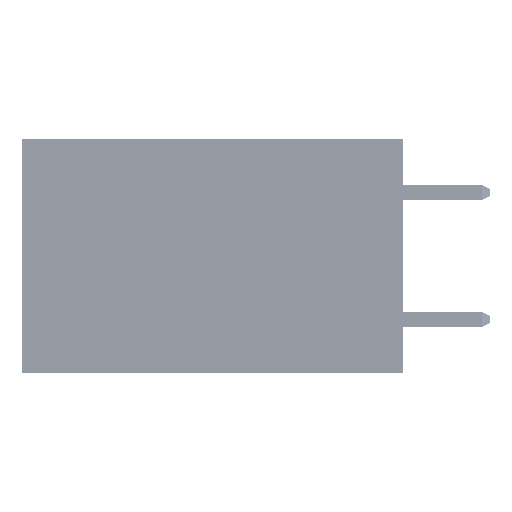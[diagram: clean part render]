
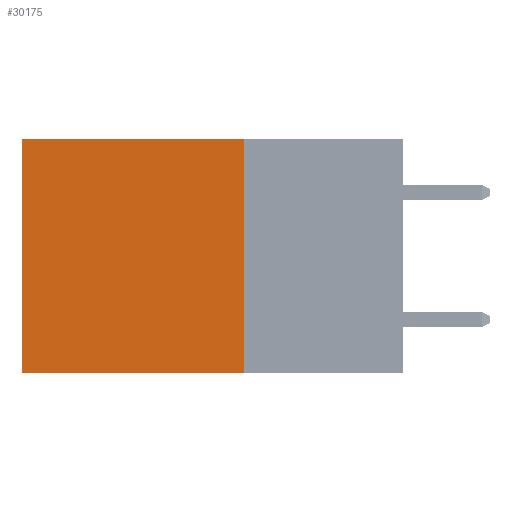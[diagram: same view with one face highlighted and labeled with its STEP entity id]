
A CAD part, left-side view. The second image highlights one B-rep face of the part: STEP entity #30175.
In plain terms, the highlighted planar face has unit normal (-1, 0, 0).
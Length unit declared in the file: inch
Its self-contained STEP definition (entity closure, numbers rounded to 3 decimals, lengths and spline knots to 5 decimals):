
#107 = ORIENTED_EDGE ( 'NONE', *, *, #25879, .F. ) ;
#2100 = CARTESIAN_POINT ( 'NONE',  ( 0.2875, 0.25, 0. ) ) ;
#3534 = VECTOR ( 'NONE', #37417, 39.37008 ) ;
#4212 = VECTOR ( 'NONE', #29039, 39.37008 ) ;
#8453 = CARTESIAN_POINT ( 'NONE',  ( 0.2875, 0.25, 0. ) ) ;
#9466 = AXIS2_PLACEMENT_3D ( 'NONE', #8453, #27998, #39258 ) ;
#11330 = VERTEX_POINT ( 'NONE', #11415 ) ;
#11401 = VERTEX_POINT ( 'NONE', #26607 ) ;
#11415 = CARTESIAN_POINT ( 'NONE',  ( 0.2875, 0.6, 0. ) ) ;
#12423 = EDGE_CURVE ( 'NONE', #17834, #11330, #48236, .T. ) ;
#12526 = CARTESIAN_POINT ( 'NONE',  ( 0.2875, 0.25, -0.37 ) ) ;
#13076 = VERTEX_POINT ( 'NONE', #12526 ) ;
#13215 = EDGE_CURVE ( 'NONE', #11330, #11401, #39036, .T. ) ;
#14314 = DIRECTION ( 'NONE',  ( 0., 0., -1. ) ) ;
#15822 = CARTESIAN_POINT ( 'NONE',  ( 0.2875, 0.25, -0.37 ) ) ;
#17834 = VERTEX_POINT ( 'NONE', #34041 ) ;
#19723 = LINE ( 'NONE', #49235, #35392 ) ;
#19757 = PLANE ( 'NONE',  #9466 ) ;
#19810 = FACE_OUTER_BOUND ( 'NONE', #33531, .T. ) ;
#24456 = ORIENTED_EDGE ( 'NONE', *, *, #12423, .T. ) ;
#25698 = ORIENTED_EDGE ( 'NONE', *, *, #13215, .T. ) ;
#25879 = EDGE_CURVE ( 'NONE', #13076, #11401, #29093, .T. ) ;
#26607 = CARTESIAN_POINT ( 'NONE',  ( 0.2875, 0.6, -0.37 ) ) ;
#27998 = DIRECTION ( 'NONE',  ( 1., 0., 0. ) ) ;
#29039 = DIRECTION ( 'NONE',  ( 0., 1., 0. ) ) ;
#29093 = LINE ( 'NONE', #15822, #38110 ) ;
#30175 = ADVANCED_FACE ( 'NONE', ( #19810 ), #19757, .F. ) ;
#30214 = ORIENTED_EDGE ( 'NONE', *, *, #42009, .F. ) ;
#33531 = EDGE_LOOP ( 'NONE', ( #25698, #107, #30214, #24456 ) ) ;
#34041 = CARTESIAN_POINT ( 'NONE',  ( 0.2875, 0.25, 0. ) ) ;
#35063 = DIRECTION ( 'NONE',  ( 0., 1., 0. ) ) ;
#35392 = VECTOR ( 'NONE', #14314, 39.37008 ) ;
#37417 = DIRECTION ( 'NONE',  ( 0., 0., -1. ) ) ;
#38110 = VECTOR ( 'NONE', #35063, 39.37008 ) ;
#39036 = LINE ( 'NONE', #48909, #3534 ) ;
#39258 = DIRECTION ( 'NONE',  ( 0., 0., -1. ) ) ;
#42009 = EDGE_CURVE ( 'NONE', #17834, #13076, #19723, .T. ) ;
#48236 = LINE ( 'NONE', #2100, #4212 ) ;
#48909 = CARTESIAN_POINT ( 'NONE',  ( 0.2875, 0.6, 0. ) ) ;
#49235 = CARTESIAN_POINT ( 'NONE',  ( 0.2875, 0.25, 0. ) ) ;
